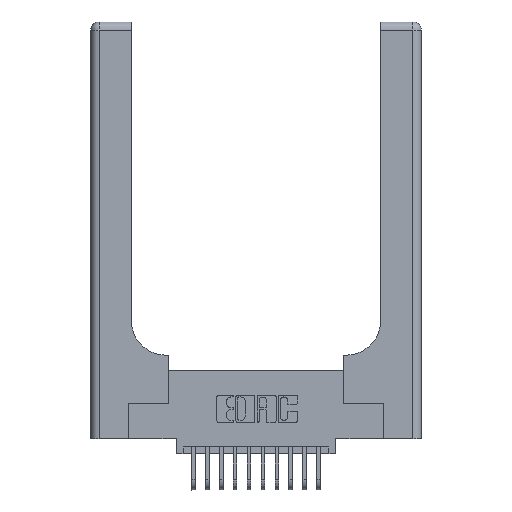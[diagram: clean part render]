
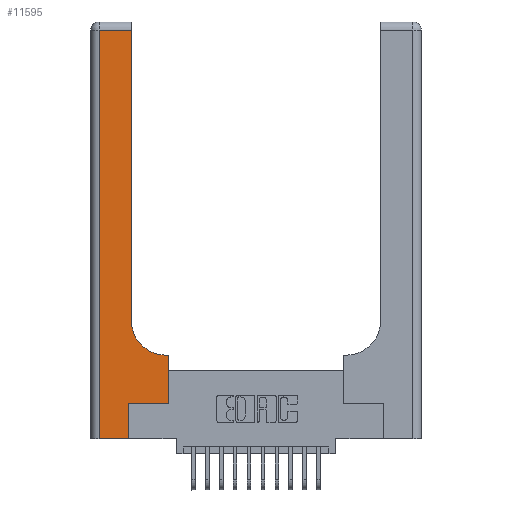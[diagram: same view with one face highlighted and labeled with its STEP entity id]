
A CAD part, top view. The second image highlights one B-rep face of the part: STEP entity #11595.
In plain terms, the highlighted planar face has unit normal (0, 0, 1).
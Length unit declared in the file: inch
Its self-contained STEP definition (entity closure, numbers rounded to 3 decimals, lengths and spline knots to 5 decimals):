
#99 = PLANE ( 'NONE',  #4615 ) ;
#182 = CARTESIAN_POINT ( 'NONE',  ( 0.5585, 0.25, 0.37 ) ) ;
#247 = CARTESIAN_POINT ( 'NONE',  ( 0.5415, 0.85, 0.37 ) ) ;
#442 = VERTEX_POINT ( 'NONE', #14888 ) ;
#624 = EDGE_LOOP ( 'NONE', ( #2988, #11327, #14795, #3245, #8384, #4299, #2048, #9262, #6066 ) ) ;
#991 = CARTESIAN_POINT ( 'NONE',  ( 0.2915, 0.85, 0.37 ) ) ;
#1683 = DIRECTION ( 'NONE',  ( 1., 0., 0. ) ) ;
#2048 = ORIENTED_EDGE ( 'NONE', *, *, #8752, .T. ) ;
#2121 = LINE ( 'NONE', #12998, #12387 ) ;
#2827 = EDGE_CURVE ( 'NONE', #7040, #6121, #7065, .T. ) ;
#2921 = DIRECTION ( 'NONE',  ( -1., 0., 0. ) ) ;
#2988 = ORIENTED_EDGE ( 'NONE', *, *, #15658, .T. ) ;
#3140 = EDGE_CURVE ( 'NONE', #3956, #6718, #9940, .T. ) ;
#3242 = VECTOR ( 'NONE', #9730, 39.37008 ) ;
#3245 = ORIENTED_EDGE ( 'NONE', *, *, #16030, .T. ) ;
#3467 = VERTEX_POINT ( 'NONE', #16827 ) ;
#3784 = CARTESIAN_POINT ( 'NONE',  ( 0.2915, 3., 0.37 ) ) ;
#3935 = VERTEX_POINT ( 'NONE', #8855 ) ;
#3937 = CARTESIAN_POINT ( 'NONE',  ( 0.269, 0., 0.37 ) ) ;
#3956 = VERTEX_POINT ( 'NONE', #4933 ) ;
#4016 = VECTOR ( 'NONE', #5349, 39.37008 ) ;
#4109 = VERTEX_POINT ( 'NONE', #5220 ) ;
#4299 = ORIENTED_EDGE ( 'NONE', *, *, #2827, .T. ) ;
#4362 = DIRECTION ( 'NONE',  ( 0., -1., 0. ) ) ;
#4615 = AXIS2_PLACEMENT_3D ( 'NONE', #9662, #10970, #2921 ) ;
#4933 = CARTESIAN_POINT ( 'NONE',  ( 0.06, 2.94, 0.37 ) ) ;
#5220 = CARTESIAN_POINT ( 'NONE',  ( 0.2915, 2.94, 0.37 ) ) ;
#5235 = DIRECTION ( 'NONE',  ( -1., 0., 0. ) ) ;
#5293 = AXIS2_PLACEMENT_3D ( 'NONE', #247, #9789, #1683 ) ;
#5349 = DIRECTION ( 'NONE',  ( 0., 1., 0. ) ) ;
#6066 = ORIENTED_EDGE ( 'NONE', *, *, #13523, .T. ) ;
#6121 = VERTEX_POINT ( 'NONE', #7583 ) ;
#6309 = EDGE_CURVE ( 'NONE', #3935, #7040, #14167, .T. ) ;
#6614 = CARTESIAN_POINT ( 'NONE',  ( 0., 2.94, 0.37 ) ) ;
#6718 = VERTEX_POINT ( 'NONE', #15315 ) ;
#6889 = LINE ( 'NONE', #182, #3242 ) ;
#7040 = VERTEX_POINT ( 'NONE', #11017 ) ;
#7065 = LINE ( 'NONE', #11745, #13640 ) ;
#7505 = VECTOR ( 'NONE', #5235, 39.37008 ) ;
#7583 = CARTESIAN_POINT ( 'NONE',  ( 0.5585, 0.25, 0.37 ) ) ;
#8333 = CARTESIAN_POINT ( 'NONE',  ( 0.06, 3., 0.37 ) ) ;
#8384 = ORIENTED_EDGE ( 'NONE', *, *, #6309, .T. ) ;
#8477 = LINE ( 'NONE', #3784, #11578 ) ;
#8552 = EDGE_CURVE ( 'NONE', #3467, #442, #12023, .T. ) ;
#8580 = EDGE_CURVE ( 'NONE', #4109, #3956, #13676, .T. ) ;
#8752 = EDGE_CURVE ( 'NONE', #6121, #3467, #6889, .T. ) ;
#8855 = CARTESIAN_POINT ( 'NONE',  ( 0.269, 0., 0.37 ) ) ;
#9113 = VERTEX_POINT ( 'NONE', #991 ) ;
#9262 = ORIENTED_EDGE ( 'NONE', *, *, #8552, .T. ) ;
#9662 = CARTESIAN_POINT ( 'NONE',  ( 0., 3., 0.37 ) ) ;
#9730 = DIRECTION ( 'NONE',  ( 0., 1., 0. ) ) ;
#9789 = DIRECTION ( 'NONE',  ( 0., 0., -1. ) ) ;
#9940 = LINE ( 'NONE', #8333, #12611 ) ;
#10456 = CARTESIAN_POINT ( 'NONE',  ( 0.2915, 0.6, 0.37 ) ) ;
#10970 = DIRECTION ( 'NONE',  ( 0., 0., -1. ) ) ;
#11017 = CARTESIAN_POINT ( 'NONE',  ( 0.269, 0.25, 0.37 ) ) ;
#11327 = ORIENTED_EDGE ( 'NONE', *, *, #8580, .T. ) ;
#11578 = VECTOR ( 'NONE', #13074, 39.37008 ) ;
#11595 = ADVANCED_FACE ( 'NONE', ( #14361 ), #99, .F. ) ;
#11745 = CARTESIAN_POINT ( 'NONE',  ( 0.269, 0.25, 0.37 ) ) ;
#12023 = LINE ( 'NONE', #10456, #7505 ) ;
#12387 = VECTOR ( 'NONE', #15561, 39.37008 ) ;
#12611 = VECTOR ( 'NONE', #4362, 39.37008 ) ;
#12998 = CARTESIAN_POINT ( 'NONE',  ( 0., 0., 0.37 ) ) ;
#13070 = DIRECTION ( 'NONE',  ( 1., 0., 0. ) ) ;
#13074 = DIRECTION ( 'NONE',  ( 0., 1., 0. ) ) ;
#13270 = VECTOR ( 'NONE', #16989, 39.37008 ) ;
#13523 = EDGE_CURVE ( 'NONE', #442, #9113, #16085, .T. ) ;
#13640 = VECTOR ( 'NONE', #13070, 39.37008 ) ;
#13676 = LINE ( 'NONE', #6614, #13270 ) ;
#14167 = LINE ( 'NONE', #3937, #4016 ) ;
#14361 = FACE_OUTER_BOUND ( 'NONE', #624, .T. ) ;
#14795 = ORIENTED_EDGE ( 'NONE', *, *, #3140, .T. ) ;
#14888 = CARTESIAN_POINT ( 'NONE',  ( 0.5415, 0.6, 0.37 ) ) ;
#15315 = CARTESIAN_POINT ( 'NONE',  ( 0.06, 0., 0.37 ) ) ;
#15561 = DIRECTION ( 'NONE',  ( 1., 0., 0. ) ) ;
#15658 = EDGE_CURVE ( 'NONE', #9113, #4109, #8477, .T. ) ;
#16030 = EDGE_CURVE ( 'NONE', #6718, #3935, #2121, .T. ) ;
#16085 = CIRCLE ( 'NONE', #5293, 0.25 ) ;
#16827 = CARTESIAN_POINT ( 'NONE',  ( 0.5585, 0.6, 0.37 ) ) ;
#16989 = DIRECTION ( 'NONE',  ( -1., 0., 0. ) ) ;
